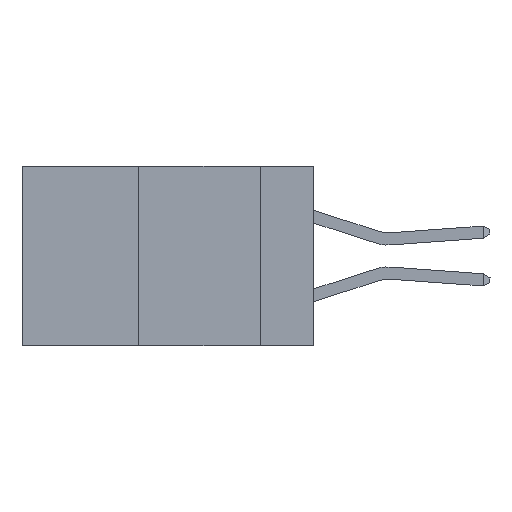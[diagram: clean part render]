
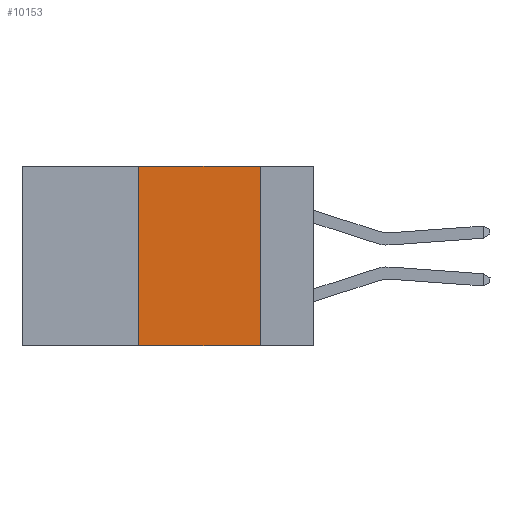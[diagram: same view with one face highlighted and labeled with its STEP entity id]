
A CAD part, left-side view. The second image highlights one B-rep face of the part: STEP entity #10153.
In plain terms, the highlighted planar face has unit normal (-1, 0, 0).
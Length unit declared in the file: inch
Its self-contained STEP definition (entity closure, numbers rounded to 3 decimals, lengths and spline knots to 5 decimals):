
#2210 = EDGE_LOOP ( 'NONE', ( #22671, #22643, #3923, #15720 ) ) ;
#3236 = VECTOR ( 'NONE', #18865, 39.37008 ) ;
#3923 = ORIENTED_EDGE ( 'NONE', *, *, #15987, .F. ) ;
#4638 = VECTOR ( 'NONE', #12247, 39.37008 ) ;
#7221 = VECTOR ( 'NONE', #23773, 39.37008 ) ;
#7323 = CARTESIAN_POINT ( 'NONE',  ( 0., 0.11, 0. ) ) ;
#8650 = CARTESIAN_POINT ( 'NONE',  ( 0., 0.36, 0. ) ) ;
#9870 = CARTESIAN_POINT ( 'NONE',  ( 0., 0.6, 0. ) ) ;
#10153 = ADVANCED_FACE ( 'NONE', ( #18222 ), #19295, .F. ) ;
#10186 = CARTESIAN_POINT ( 'NONE',  ( 0., 0.6, 0. ) ) ;
#10194 = DIRECTION ( 'NONE',  ( 0., 0., -1. ) ) ;
#10967 = VERTEX_POINT ( 'NONE', #15851 ) ;
#11130 = CARTESIAN_POINT ( 'NONE',  ( 0., 0.6, -0.37 ) ) ;
#11234 = VERTEX_POINT ( 'NONE', #16590 ) ;
#12247 = DIRECTION ( 'NONE',  ( 0., -1., 0. ) ) ;
#12504 = LINE ( 'NONE', #11130, #3236 ) ;
#12660 = VECTOR ( 'NONE', #17078, 39.37008 ) ;
#12783 = EDGE_CURVE ( 'NONE', #23832, #23467, #14262, .T. ) ;
#13883 = DIRECTION ( 'NONE',  ( 1., 0., 0. ) ) ;
#14262 = LINE ( 'NONE', #10186, #4638 ) ;
#15720 = ORIENTED_EDGE ( 'NONE', *, *, #17553, .T. ) ;
#15851 = CARTESIAN_POINT ( 'NONE',  ( 0., 0.11, -0.37 ) ) ;
#15987 = EDGE_CURVE ( 'NONE', #11234, #23832, #19489, .T. ) ;
#16590 = CARTESIAN_POINT ( 'NONE',  ( 0., 0.36, -0.37 ) ) ;
#17044 = AXIS2_PLACEMENT_3D ( 'NONE', #9870, #13883, #10194 ) ;
#17078 = DIRECTION ( 'NONE',  ( 0., 0., -1. ) ) ;
#17553 = EDGE_CURVE ( 'NONE', #11234, #10967, #12504, .T. ) ;
#17785 = CARTESIAN_POINT ( 'NONE',  ( 0., 0.36, 0. ) ) ;
#18222 = FACE_OUTER_BOUND ( 'NONE', #2210, .T. ) ;
#18816 = CARTESIAN_POINT ( 'NONE',  ( 0., 0.11, 0. ) ) ;
#18865 = DIRECTION ( 'NONE',  ( 0., -1., 0. ) ) ;
#19295 = PLANE ( 'NONE',  #17044 ) ;
#19489 = LINE ( 'NONE', #17785, #7221 ) ;
#22530 = LINE ( 'NONE', #18816, #12660 ) ;
#22643 = ORIENTED_EDGE ( 'NONE', *, *, #12783, .F. ) ;
#22671 = ORIENTED_EDGE ( 'NONE', *, *, #24161, .F. ) ;
#23467 = VERTEX_POINT ( 'NONE', #7323 ) ;
#23773 = DIRECTION ( 'NONE',  ( 0., 0., 1. ) ) ;
#23832 = VERTEX_POINT ( 'NONE', #8650 ) ;
#24161 = EDGE_CURVE ( 'NONE', #23467, #10967, #22530, .T. ) ;
